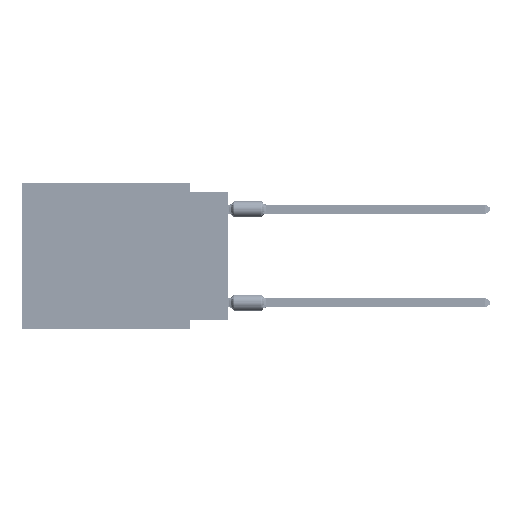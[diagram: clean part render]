
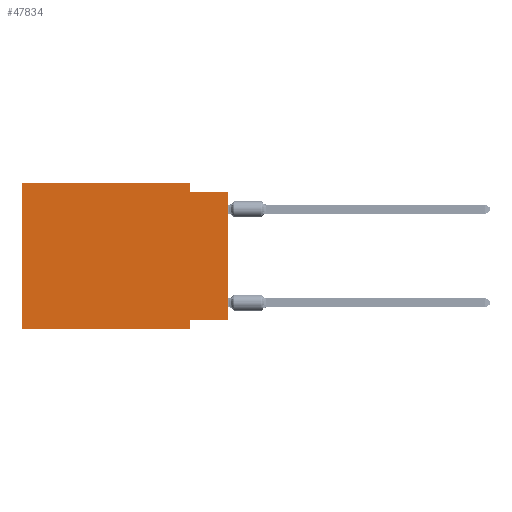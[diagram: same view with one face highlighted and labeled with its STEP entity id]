
A CAD part, left-side view. The second image highlights one B-rep face of the part: STEP entity #47834.
In plain terms, the highlighted planar face has unit normal (-1, 0, 0).
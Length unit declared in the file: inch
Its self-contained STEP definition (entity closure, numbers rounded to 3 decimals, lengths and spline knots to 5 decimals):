
#3052 = VECTOR ( 'NONE', #46076, 39.37008 ) ;
#3806 = CARTESIAN_POINT ( 'NONE',  ( 0., 0.1, -0.39 ) ) ;
#3936 = CARTESIAN_POINT ( 'NONE',  ( 0., 0.55, 0. ) ) ;
#4111 = LINE ( 'NONE', #30581, #31384 ) ;
#4488 = DIRECTION ( 'NONE',  ( 0., 0., -1. ) ) ;
#6410 = ORIENTED_EDGE ( 'NONE', *, *, #74319, .F. ) ;
#7363 = DIRECTION ( 'NONE',  ( 0., 0., 1. ) ) ;
#7832 = VERTEX_POINT ( 'NONE', #3936 ) ;
#8883 = CARTESIAN_POINT ( 'NONE',  ( 0., 0., -0.025 ) ) ;
#10592 = FACE_OUTER_BOUND ( 'NONE', #34355, .T. ) ;
#11006 = CARTESIAN_POINT ( 'NONE',  ( 0., 0.55, 0. ) ) ;
#12020 = EDGE_CURVE ( 'NONE', #47799, #79572, #36749, .T. ) ;
#12924 = VECTOR ( 'NONE', #43700, 39.37008 ) ;
#13774 = VERTEX_POINT ( 'NONE', #48542 ) ;
#16417 = DIRECTION ( 'NONE',  ( 0., 0., -1. ) ) ;
#16720 = DIRECTION ( 'NONE',  ( 0., -1., 0. ) ) ;
#18898 = EDGE_CURVE ( 'NONE', #21126, #7832, #40344, .T. ) ;
#19573 = CARTESIAN_POINT ( 'NONE',  ( 0., 0., -0.365 ) ) ;
#21126 = VERTEX_POINT ( 'NONE', #47472 ) ;
#23185 = ORIENTED_EDGE ( 'NONE', *, *, #18898, .F. ) ;
#25632 = LINE ( 'NONE', #78625, #56094 ) ;
#29644 = ORIENTED_EDGE ( 'NONE', *, *, #36420, .F. ) ;
#30136 = VECTOR ( 'NONE', #16417, 39.37008 ) ;
#30581 = CARTESIAN_POINT ( 'NONE',  ( 0., 0.55, -0.39 ) ) ;
#31384 = VECTOR ( 'NONE', #16720, 39.37008 ) ;
#32602 = EDGE_CURVE ( 'NONE', #13774, #34108, #25632, .T. ) ;
#33678 = EDGE_CURVE ( 'NONE', #34108, #79572, #50868, .T. ) ;
#33830 = CARTESIAN_POINT ( 'NONE',  ( 0., 0.55, 0. ) ) ;
#34108 = VERTEX_POINT ( 'NONE', #57272 ) ;
#34355 = EDGE_LOOP ( 'NONE', ( #49557, #84857, #70887, #29644, #23185, #60003, #6410, #41772 ) ) ;
#36420 = EDGE_CURVE ( 'NONE', #7832, #13774, #46886, .T. ) ;
#36749 = LINE ( 'NONE', #83632, #12924 ) ;
#37051 = PLANE ( 'NONE',  #83989 ) ;
#37462 = CARTESIAN_POINT ( 'NONE',  ( 0., 0., -0.365 ) ) ;
#39381 = CARTESIAN_POINT ( 'NONE',  ( 0., 0.1, -0.39 ) ) ;
#40344 = LINE ( 'NONE', #66868, #77622 ) ;
#41772 = ORIENTED_EDGE ( 'NONE', *, *, #81732, .F. ) ;
#43498 = CARTESIAN_POINT ( 'NONE',  ( 0., 0., -0.025 ) ) ;
#43700 = DIRECTION ( 'NONE',  ( 0., 0., 1. ) ) ;
#44331 = DIRECTION ( 'NONE',  ( 0., 0., -1. ) ) ;
#46076 = DIRECTION ( 'NONE',  ( 0., 1., 0. ) ) ;
#46886 = LINE ( 'NONE', #33830, #85697 ) ;
#47472 = CARTESIAN_POINT ( 'NONE',  ( 0., 0.55, -0.39 ) ) ;
#47799 = VERTEX_POINT ( 'NONE', #37462 ) ;
#47834 = ADVANCED_FACE ( 'NONE', ( #10592 ), #37051, .F. ) ;
#48348 = VERTEX_POINT ( 'NONE', #39381 ) ;
#48542 = CARTESIAN_POINT ( 'NONE',  ( 0., 0.1, 0. ) ) ;
#49178 = DIRECTION ( 'NONE',  ( 0., -1., 0. ) ) ;
#49557 = ORIENTED_EDGE ( 'NONE', *, *, #12020, .T. ) ;
#50868 = LINE ( 'NONE', #43498, #78390 ) ;
#56094 = VECTOR ( 'NONE', #44331, 39.37008 ) ;
#57272 = CARTESIAN_POINT ( 'NONE',  ( 0., 0.1, -0.025 ) ) ;
#60003 = ORIENTED_EDGE ( 'NONE', *, *, #73028, .T. ) ;
#62275 = VERTEX_POINT ( 'NONE', #84812 ) ;
#62898 = LINE ( 'NONE', #3806, #30136 ) ;
#64001 = DIRECTION ( 'NONE',  ( 1., 0., 0. ) ) ;
#66868 = CARTESIAN_POINT ( 'NONE',  ( 0., 0.55, 0. ) ) ;
#67296 = DIRECTION ( 'NONE',  ( 0., -1., 0. ) ) ;
#68975 = LINE ( 'NONE', #19573, #3052 ) ;
#70887 = ORIENTED_EDGE ( 'NONE', *, *, #32602, .F. ) ;
#73028 = EDGE_CURVE ( 'NONE', #21126, #48348, #4111, .T. ) ;
#74319 = EDGE_CURVE ( 'NONE', #62275, #48348, #62898, .T. ) ;
#77622 = VECTOR ( 'NONE', #7363, 39.37008 ) ;
#78390 = VECTOR ( 'NONE', #49178, 39.37008 ) ;
#78625 = CARTESIAN_POINT ( 'NONE',  ( 0., 0.1, 0. ) ) ;
#79572 = VERTEX_POINT ( 'NONE', #8883 ) ;
#81732 = EDGE_CURVE ( 'NONE', #47799, #62275, #68975, .T. ) ;
#83632 = CARTESIAN_POINT ( 'NONE',  ( 0., 0., 0. ) ) ;
#83989 = AXIS2_PLACEMENT_3D ( 'NONE', #11006, #64001, #4488 ) ;
#84812 = CARTESIAN_POINT ( 'NONE',  ( 0., 0.1, -0.365 ) ) ;
#84857 = ORIENTED_EDGE ( 'NONE', *, *, #33678, .F. ) ;
#85697 = VECTOR ( 'NONE', #67296, 39.37008 ) ;
